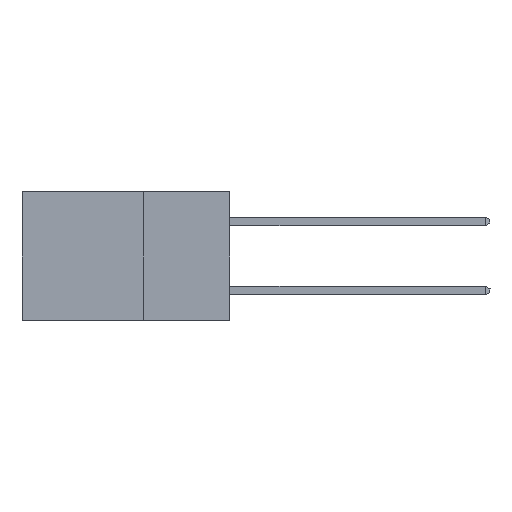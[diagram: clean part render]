
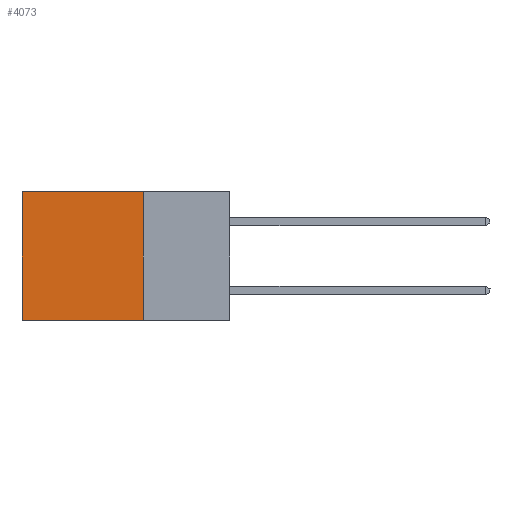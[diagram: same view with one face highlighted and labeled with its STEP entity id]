
A CAD part, left-side view. The second image highlights one B-rep face of the part: STEP entity #4073.
In plain terms, the highlighted planar face has unit normal (-1, 0, 0).
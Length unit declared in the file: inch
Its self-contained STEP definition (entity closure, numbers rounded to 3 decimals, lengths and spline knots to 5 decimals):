
#481 = LINE ( 'NONE', #18616, #16231 ) ;
#1954 = CARTESIAN_POINT ( 'NONE',  ( 0.2615, 0.25, -0.37 ) ) ;
#2308 = CARTESIAN_POINT ( 'NONE',  ( 0.2615, 0.25, 0. ) ) ;
#4013 = EDGE_CURVE ( 'NONE', #16424, #5029, #7006, .T. ) ;
#4073 = ADVANCED_FACE ( 'NONE', ( #10660 ), #20259, .F. ) ;
#5029 = VERTEX_POINT ( 'NONE', #25199 ) ;
#5276 = CARTESIAN_POINT ( 'NONE',  ( 0.2615, 0.25, -0.37 ) ) ;
#5809 = VERTEX_POINT ( 'NONE', #2308 ) ;
#6327 = EDGE_CURVE ( 'NONE', #5809, #20314, #481, .T. ) ;
#7006 = LINE ( 'NONE', #5276, #17652 ) ;
#8032 = DIRECTION ( 'NONE',  ( 0., 1., 0. ) ) ;
#8423 = CARTESIAN_POINT ( 'NONE',  ( 0.2615, 0.6, 0. ) ) ;
#10660 = FACE_OUTER_BOUND ( 'NONE', #19883, .T. ) ;
#10947 = DIRECTION ( 'NONE',  ( 0., 0., -1. ) ) ;
#13424 = ORIENTED_EDGE ( 'NONE', *, *, #4013, .F. ) ;
#14065 = DIRECTION ( 'NONE',  ( 0., 0., -1. ) ) ;
#15908 = DIRECTION ( 'NONE',  ( 0., 1., 0. ) ) ;
#16231 = VECTOR ( 'NONE', #8032, 39.37008 ) ;
#16275 = CARTESIAN_POINT ( 'NONE',  ( 0.2615, 0.25, -0.37 ) ) ;
#16424 = VERTEX_POINT ( 'NONE', #16275 ) ;
#16562 = LINE ( 'NONE', #23544, #17230 ) ;
#16987 = ORIENTED_EDGE ( 'NONE', *, *, #19369, .F. ) ;
#17230 = VECTOR ( 'NONE', #10947, 39.37008 ) ;
#17652 = VECTOR ( 'NONE', #15908, 39.37008 ) ;
#18616 = CARTESIAN_POINT ( 'NONE',  ( 0.2615, 0.25, 0. ) ) ;
#19369 = EDGE_CURVE ( 'NONE', #5809, #16424, #26429, .T. ) ;
#19883 = EDGE_LOOP ( 'NONE', ( #26273, #13424, #16987, #21852 ) ) ;
#20259 = PLANE ( 'NONE',  #22446 ) ;
#20314 = VERTEX_POINT ( 'NONE', #8423 ) ;
#21579 = VECTOR ( 'NONE', #23156, 39.37008 ) ;
#21852 = ORIENTED_EDGE ( 'NONE', *, *, #6327, .T. ) ;
#22446 = AXIS2_PLACEMENT_3D ( 'NONE', #24464, #26510, #14065 ) ;
#23156 = DIRECTION ( 'NONE',  ( 0., 0., -1. ) ) ;
#23544 = CARTESIAN_POINT ( 'NONE',  ( 0.2615, 0.6, -0.37 ) ) ;
#23649 = EDGE_CURVE ( 'NONE', #20314, #5029, #16562, .T. ) ;
#24464 = CARTESIAN_POINT ( 'NONE',  ( 0.2615, 0.25, -0.37 ) ) ;
#25199 = CARTESIAN_POINT ( 'NONE',  ( 0.2615, 0.6, -0.37 ) ) ;
#26273 = ORIENTED_EDGE ( 'NONE', *, *, #23649, .T. ) ;
#26429 = LINE ( 'NONE', #1954, #21579 ) ;
#26510 = DIRECTION ( 'NONE',  ( 1., 0., 0. ) ) ;
